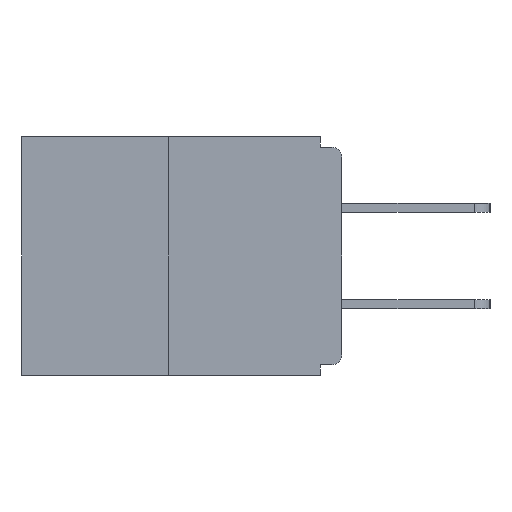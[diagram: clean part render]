
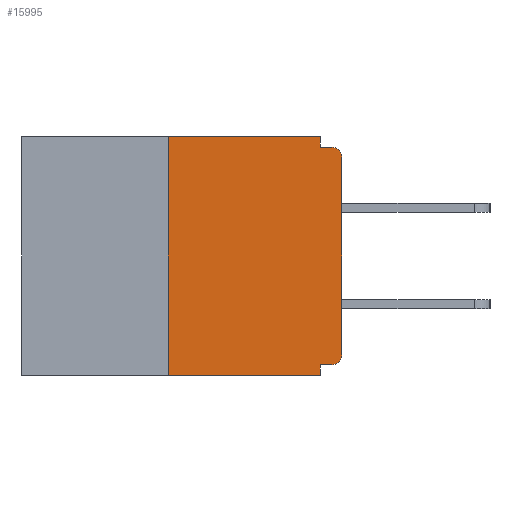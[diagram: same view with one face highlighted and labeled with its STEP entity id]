
A CAD part, left-side view. The second image highlights one B-rep face of the part: STEP entity #15995.
In plain terms, the highlighted planar face has unit normal (-1, 0, 0).
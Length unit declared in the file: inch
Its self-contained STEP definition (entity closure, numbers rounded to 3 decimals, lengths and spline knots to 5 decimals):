
#152 = ORIENTED_EDGE ( 'NONE', *, *, #3957, .F. ) ;
#163 = DIRECTION ( 'NONE',  ( -1., 0., 0. ) ) ;
#671 = LINE ( 'NONE', #9709, #13032 ) ;
#1080 = PLANE ( 'NONE',  #1630 ) ;
#1159 = VERTEX_POINT ( 'NONE', #8951 ) ;
#1235 = EDGE_CURVE ( 'NONE', #1932, #12212, #15297, .T. ) ;
#1630 = AXIS2_PLACEMENT_3D ( 'NONE', #14682, #9990, #3903 ) ;
#1648 = DIRECTION ( 'NONE',  ( 0., 0., -1. ) ) ;
#1694 = CARTESIAN_POINT ( 'NONE',  ( 0., 0.015, -0.313 ) ) ;
#1871 = LINE ( 'NONE', #14901, #12104 ) ;
#1924 = VECTOR ( 'NONE', #5042, 39.37008 ) ;
#1932 = VERTEX_POINT ( 'NONE', #3971 ) ;
#2031 = FACE_OUTER_BOUND ( 'NONE', #4738, .T. ) ;
#2173 = EDGE_CURVE ( 'NONE', #15797, #4735, #3169, .T. ) ;
#2406 = AXIS2_PLACEMENT_3D ( 'NONE', #8667, #13198, #13321 ) ;
#2758 = VECTOR ( 'NONE', #1648, 39.37008 ) ;
#3169 = CIRCLE ( 'NONE', #18739, 0.015 ) ;
#3373 = CARTESIAN_POINT ( 'NONE',  ( 0., 0.031, -0.328 ) ) ;
#3813 = VERTEX_POINT ( 'NONE', #11835 ) ;
#3903 = DIRECTION ( 'NONE',  ( 0., 0., -1. ) ) ;
#3957 = EDGE_CURVE ( 'NONE', #4530, #1932, #5015, .T. ) ;
#3971 = CARTESIAN_POINT ( 'NONE',  ( 0., 0.031, -0.015 ) ) ;
#4530 = VERTEX_POINT ( 'NONE', #19098 ) ;
#4735 = VERTEX_POINT ( 'NONE', #10899 ) ;
#4738 = EDGE_LOOP ( 'NONE', ( #14162, #7482, #10870, #16395, #17467, #13283, #18265, #6055, #6875, #152 ) ) ;
#5015 = LINE ( 'NONE', #6447, #1924 ) ;
#5042 = DIRECTION ( 'NONE',  ( 0., 0., -1. ) ) ;
#5252 = EDGE_CURVE ( 'NONE', #1159, #3813, #1871, .T. ) ;
#6055 = ORIENTED_EDGE ( 'NONE', *, *, #7157, .T. ) ;
#6127 = LINE ( 'NONE', #6185, #2758 ) ;
#6185 = CARTESIAN_POINT ( 'NONE',  ( 0., 0.031, -0.343 ) ) ;
#6293 = LINE ( 'NONE', #15370, #7928 ) ;
#6447 = CARTESIAN_POINT ( 'NONE',  ( 0., 0.031, 0. ) ) ;
#6875 = ORIENTED_EDGE ( 'NONE', *, *, #1235, .F. ) ;
#7157 = EDGE_CURVE ( 'NONE', #7197, #12212, #12586, .T. ) ;
#7197 = VERTEX_POINT ( 'NONE', #17798 ) ;
#7334 = DIRECTION ( 'NONE',  ( 0., 0., -1. ) ) ;
#7482 = ORIENTED_EDGE ( 'NONE', *, *, #5252, .F. ) ;
#7538 = EDGE_CURVE ( 'NONE', #4735, #7197, #671, .T. ) ;
#7928 = VECTOR ( 'NONE', #18350, 39.37008 ) ;
#8667 = CARTESIAN_POINT ( 'NONE',  ( 0., 0.015, -0.03 ) ) ;
#8864 = EDGE_CURVE ( 'NONE', #3813, #4530, #9413, .T. ) ;
#8951 = CARTESIAN_POINT ( 'NONE',  ( 0., 0.25, -0.343 ) ) ;
#9413 = LINE ( 'NONE', #11891, #14401 ) ;
#9709 = CARTESIAN_POINT ( 'NONE',  ( 0., 0., 0. ) ) ;
#9711 = VERTEX_POINT ( 'NONE', #11616 ) ;
#9736 = CARTESIAN_POINT ( 'NONE',  ( 0., 0., -0.328 ) ) ;
#9990 = DIRECTION ( 'NONE',  ( 1., 0., 0. ) ) ;
#10203 = LINE ( 'NONE', #9736, #12139 ) ;
#10870 = ORIENTED_EDGE ( 'NONE', *, *, #10949, .T. ) ;
#10899 = CARTESIAN_POINT ( 'NONE',  ( 0., 0., -0.313 ) ) ;
#10949 = EDGE_CURVE ( 'NONE', #1159, #9711, #6293, .T. ) ;
#11616 = CARTESIAN_POINT ( 'NONE',  ( 0., 0.031, -0.343 ) ) ;
#11835 = CARTESIAN_POINT ( 'NONE',  ( 0., 0.25, 0. ) ) ;
#11891 = CARTESIAN_POINT ( 'NONE',  ( 0., 0.46, 0. ) ) ;
#12092 = DIRECTION ( 'NONE',  ( 0., 0., 1. ) ) ;
#12104 = VECTOR ( 'NONE', #12092, 39.37008 ) ;
#12139 = VECTOR ( 'NONE', #14387, 39.37008 ) ;
#12212 = VERTEX_POINT ( 'NONE', #15810 ) ;
#12345 = VERTEX_POINT ( 'NONE', #3373 ) ;
#12586 = CIRCLE ( 'NONE', #2406, 0.015 ) ;
#13032 = VECTOR ( 'NONE', #17264, 39.37008 ) ;
#13198 = DIRECTION ( 'NONE',  ( -1., 0., 0. ) ) ;
#13283 = ORIENTED_EDGE ( 'NONE', *, *, #2173, .T. ) ;
#13321 = DIRECTION ( 'NONE',  ( 0., 0., -1. ) ) ;
#14162 = ORIENTED_EDGE ( 'NONE', *, *, #8864, .F. ) ;
#14387 = DIRECTION ( 'NONE',  ( 0., 1., 0. ) ) ;
#14401 = VECTOR ( 'NONE', #16518, 39.37008 ) ;
#14676 = DIRECTION ( 'NONE',  ( 0., -1., 0. ) ) ;
#14682 = CARTESIAN_POINT ( 'NONE',  ( 0., 0.46, 0. ) ) ;
#14882 = CARTESIAN_POINT ( 'NONE',  ( 0., 0., -0.015 ) ) ;
#14901 = CARTESIAN_POINT ( 'NONE',  ( 0., 0.25, 0. ) ) ;
#15114 = EDGE_CURVE ( 'NONE', #12345, #9711, #6127, .T. ) ;
#15297 = LINE ( 'NONE', #14882, #16971 ) ;
#15370 = CARTESIAN_POINT ( 'NONE',  ( 0., 0.46, -0.343 ) ) ;
#15436 = CARTESIAN_POINT ( 'NONE',  ( 0., 0.015, -0.328 ) ) ;
#15797 = VERTEX_POINT ( 'NONE', #15436 ) ;
#15810 = CARTESIAN_POINT ( 'NONE',  ( 0., 0.015, -0.015 ) ) ;
#15995 = ADVANCED_FACE ( 'NONE', ( #2031 ), #1080, .F. ) ;
#16395 = ORIENTED_EDGE ( 'NONE', *, *, #15114, .F. ) ;
#16518 = DIRECTION ( 'NONE',  ( 0., -1., 0. ) ) ;
#16971 = VECTOR ( 'NONE', #14676, 39.37008 ) ;
#17264 = DIRECTION ( 'NONE',  ( 0., 0., 1. ) ) ;
#17467 = ORIENTED_EDGE ( 'NONE', *, *, #18847, .F. ) ;
#17798 = CARTESIAN_POINT ( 'NONE',  ( 0., 0., -0.03 ) ) ;
#18265 = ORIENTED_EDGE ( 'NONE', *, *, #7538, .T. ) ;
#18350 = DIRECTION ( 'NONE',  ( 0., -1., 0. ) ) ;
#18739 = AXIS2_PLACEMENT_3D ( 'NONE', #1694, #163, #7334 ) ;
#18847 = EDGE_CURVE ( 'NONE', #15797, #12345, #10203, .T. ) ;
#19098 = CARTESIAN_POINT ( 'NONE',  ( 0., 0.031, 0. ) ) ;
